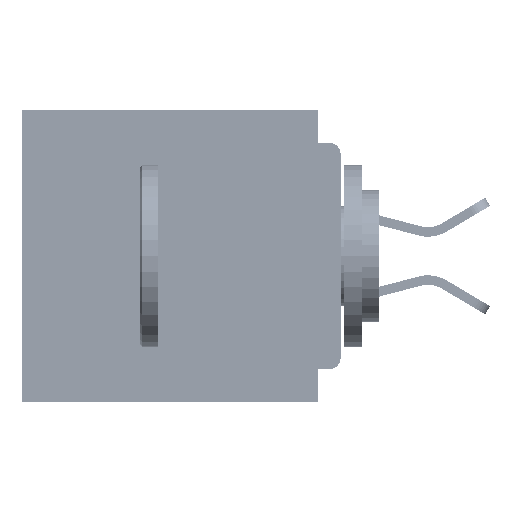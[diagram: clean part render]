
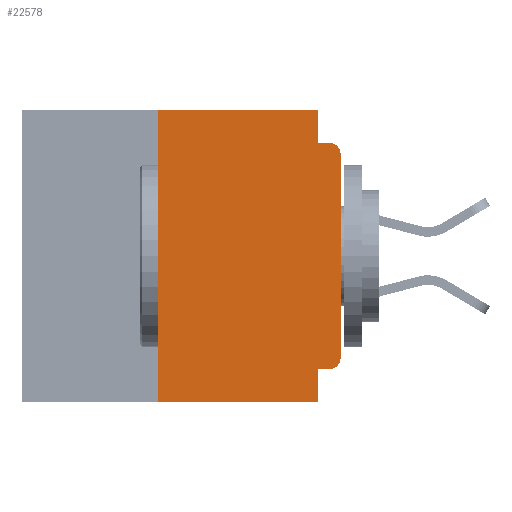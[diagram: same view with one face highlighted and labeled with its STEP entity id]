
A CAD part, left-side view. The second image highlights one B-rep face of the part: STEP entity #22578.
In plain terms, the highlighted planar face has unit normal (-1, 0, 0).
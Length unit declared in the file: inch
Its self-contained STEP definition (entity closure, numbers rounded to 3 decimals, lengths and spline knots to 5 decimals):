
#14 = VECTOR ( 'NONE', #13607, 39.37008 ) ;
#576 = VERTEX_POINT ( 'NONE', #47813 ) ;
#706 = VECTOR ( 'NONE', #46752, 39.37008 ) ;
#1487 = ORIENTED_EDGE ( 'NONE', *, *, #37870, .F. ) ;
#2567 = DIRECTION ( 'NONE',  ( 1., 0., 0. ) ) ;
#2721 = LINE ( 'NONE', #49702, #13091 ) ;
#4053 = EDGE_CURVE ( 'NONE', #15030, #6587, #10673, .T. ) ;
#4061 = DIRECTION ( 'NONE',  ( 0., -1., 0. ) ) ;
#4555 = VERTEX_POINT ( 'NONE', #28920 ) ;
#5989 = AXIS2_PLACEMENT_3D ( 'NONE', #10692, #41217, #15109 ) ;
#6587 = VERTEX_POINT ( 'NONE', #55796 ) ;
#6941 = LINE ( 'NONE', #28665, #52032 ) ;
#6999 = LINE ( 'NONE', #7860, #8373 ) ;
#7438 = AXIS2_PLACEMENT_3D ( 'NONE', #49268, #23201, #53634 ) ;
#7860 = CARTESIAN_POINT ( 'NONE',  ( 0., 0.437, -0.4 ) ) ;
#8078 = LINE ( 'NONE', #24233, #18431 ) ;
#8373 = VECTOR ( 'NONE', #34048, 39.37008 ) ;
#10426 = DIRECTION ( 'NONE',  ( 0., 0., 1. ) ) ;
#10673 = LINE ( 'NONE', #42678, #55669 ) ;
#10692 = CARTESIAN_POINT ( 'NONE',  ( 0., 0.015, -0.34 ) ) ;
#11007 = AXIS2_PLACEMENT_3D ( 'NONE', #11301, #2567, #33200 ) ;
#11133 = LINE ( 'NONE', #16285, #706 ) ;
#11301 = CARTESIAN_POINT ( 'NONE',  ( 0., 0.437, 0. ) ) ;
#11670 = ORIENTED_EDGE ( 'NONE', *, *, #15947, .F. ) ;
#13091 = VECTOR ( 'NONE', #10426, 39.37008 ) ;
#13431 = ORIENTED_EDGE ( 'NONE', *, *, #43545, .F. ) ;
#13607 = DIRECTION ( 'NONE',  ( 0., 0., -1. ) ) ;
#13865 = VERTEX_POINT ( 'NONE', #48262 ) ;
#14404 = VERTEX_POINT ( 'NONE', #44428 ) ;
#15030 = VERTEX_POINT ( 'NONE', #39947 ) ;
#15109 = DIRECTION ( 'NONE',  ( 0., 0., -1. ) ) ;
#15231 = CARTESIAN_POINT ( 'NONE',  ( 0., 0.031, -0.4 ) ) ;
#15947 = EDGE_CURVE ( 'NONE', #13865, #54678, #6941, .T. ) ;
#16285 = CARTESIAN_POINT ( 'NONE',  ( 0., 0.031, -0.4 ) ) ;
#18431 = VECTOR ( 'NONE', #50305, 39.37008 ) ;
#21488 = ORIENTED_EDGE ( 'NONE', *, *, #41871, .T. ) ;
#22383 = EDGE_CURVE ( 'NONE', #54678, #27549, #46630, .T. ) ;
#22578 = ADVANCED_FACE ( 'NONE', ( #48643 ), #54931, .F. ) ;
#22638 = EDGE_CURVE ( 'NONE', #14404, #43930, #11133, .T. ) ;
#23201 = DIRECTION ( 'NONE',  ( -1., 0., 0. ) ) ;
#24233 = CARTESIAN_POINT ( 'NONE',  ( 0., 0., -0.355 ) ) ;
#25132 = VERTEX_POINT ( 'NONE', #37961 ) ;
#27549 = VERTEX_POINT ( 'NONE', #55654 ) ;
#27756 = LINE ( 'NONE', #56377, #48155 ) ;
#28665 = CARTESIAN_POINT ( 'NONE',  ( 0., 0.437, 0. ) ) ;
#28920 = CARTESIAN_POINT ( 'NONE',  ( 0., 0.015, -0.045 ) ) ;
#29347 = CARTESIAN_POINT ( 'NONE',  ( 0., 0.031, 0. ) ) ;
#29718 = DIRECTION ( 'NONE',  ( 0., 0., 1. ) ) ;
#30504 = ORIENTED_EDGE ( 'NONE', *, *, #4053, .T. ) ;
#32979 = DIRECTION ( 'NONE',  ( 0., -1., 0. ) ) ;
#33200 = DIRECTION ( 'NONE',  ( 0., 0., -1. ) ) ;
#34048 = DIRECTION ( 'NONE',  ( 0., -1., 0. ) ) ;
#34948 = ORIENTED_EDGE ( 'NONE', *, *, #22638, .F. ) ;
#36684 = EDGE_CURVE ( 'NONE', #576, #13865, #2721, .T. ) ;
#37319 = CIRCLE ( 'NONE', #5989, 0.015 ) ;
#37870 = EDGE_CURVE ( 'NONE', #25132, #14404, #8078, .T. ) ;
#37961 = CARTESIAN_POINT ( 'NONE',  ( 0., 0.015, -0.355 ) ) ;
#39947 = CARTESIAN_POINT ( 'NONE',  ( 0., 0., -0.34 ) ) ;
#41217 = DIRECTION ( 'NONE',  ( -1., 0., 0. ) ) ;
#41871 = EDGE_CURVE ( 'NONE', #576, #43930, #6999, .T. ) ;
#42678 = CARTESIAN_POINT ( 'NONE',  ( 0., 0., 0. ) ) ;
#42905 = EDGE_CURVE ( 'NONE', #25132, #15030, #37319, .T. ) ;
#43545 = EDGE_CURVE ( 'NONE', #27549, #4555, #27756, .T. ) ;
#43930 = VERTEX_POINT ( 'NONE', #15231 ) ;
#44428 = CARTESIAN_POINT ( 'NONE',  ( 0., 0.031, -0.355 ) ) ;
#44877 = ORIENTED_EDGE ( 'NONE', *, *, #22383, .F. ) ;
#46630 = LINE ( 'NONE', #48463, #14 ) ;
#46752 = DIRECTION ( 'NONE',  ( 0., 0., -1. ) ) ;
#47813 = CARTESIAN_POINT ( 'NONE',  ( 0., 0.25, -0.4 ) ) ;
#48155 = VECTOR ( 'NONE', #4061, 39.37008 ) ;
#48262 = CARTESIAN_POINT ( 'NONE',  ( 0., 0.25, 0. ) ) ;
#48463 = CARTESIAN_POINT ( 'NONE',  ( 0., 0.031, 0. ) ) ;
#48643 = FACE_OUTER_BOUND ( 'NONE', #55490, .T. ) ;
#49268 = CARTESIAN_POINT ( 'NONE',  ( 0., 0.015, -0.06 ) ) ;
#49702 = CARTESIAN_POINT ( 'NONE',  ( 0., 0.25, -0.4 ) ) ;
#50199 = ORIENTED_EDGE ( 'NONE', *, *, #51631, .T. ) ;
#50305 = DIRECTION ( 'NONE',  ( 0., 1., 0. ) ) ;
#51631 = EDGE_CURVE ( 'NONE', #6587, #4555, #54209, .T. ) ;
#52032 = VECTOR ( 'NONE', #32979, 39.37008 ) ;
#52450 = ORIENTED_EDGE ( 'NONE', *, *, #42905, .T. ) ;
#52768 = ORIENTED_EDGE ( 'NONE', *, *, #36684, .F. ) ;
#53634 = DIRECTION ( 'NONE',  ( 0., 0., -1. ) ) ;
#54209 = CIRCLE ( 'NONE', #7438, 0.015 ) ;
#54678 = VERTEX_POINT ( 'NONE', #29347 ) ;
#54931 = PLANE ( 'NONE',  #11007 ) ;
#55490 = EDGE_LOOP ( 'NONE', ( #30504, #50199, #13431, #44877, #11670, #52768, #21488, #34948, #1487, #52450 ) ) ;
#55654 = CARTESIAN_POINT ( 'NONE',  ( 0., 0.031, -0.045 ) ) ;
#55669 = VECTOR ( 'NONE', #29718, 39.37008 ) ;
#55796 = CARTESIAN_POINT ( 'NONE',  ( 0., 0., -0.06 ) ) ;
#56377 = CARTESIAN_POINT ( 'NONE',  ( 0., 0., -0.045 ) ) ;
